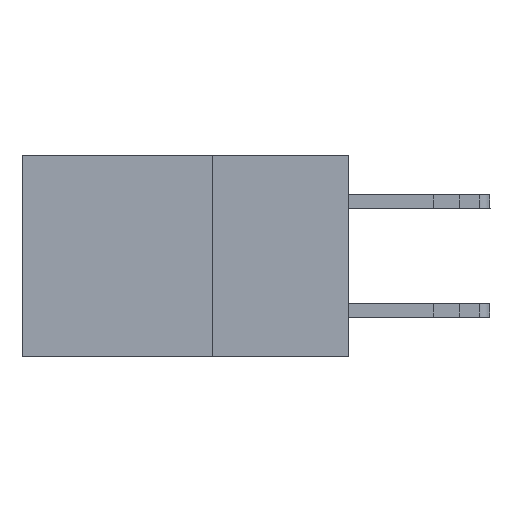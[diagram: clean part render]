
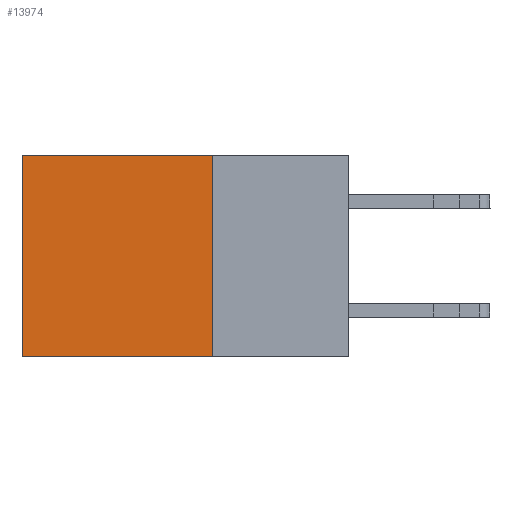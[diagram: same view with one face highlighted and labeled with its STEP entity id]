
A CAD part, left-side view. The second image highlights one B-rep face of the part: STEP entity #13974.
In plain terms, the highlighted planar face has unit normal (-1, 0, 0).
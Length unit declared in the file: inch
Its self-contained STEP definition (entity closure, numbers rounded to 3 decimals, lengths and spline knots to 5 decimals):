
#588 = FACE_OUTER_BOUND ( 'NONE', #6621, .T. ) ;
#638 = CARTESIAN_POINT ( 'NONE',  ( 0.2615, 0.25, -0.37 ) ) ;
#677 = VERTEX_POINT ( 'NONE', #7158 ) ;
#799 = DIRECTION ( 'NONE',  ( 0., 1., 0. ) ) ;
#973 = VECTOR ( 'NONE', #9903, 39.37008 ) ;
#1036 = VERTEX_POINT ( 'NONE', #10401 ) ;
#1216 = VERTEX_POINT ( 'NONE', #12001 ) ;
#2513 = DIRECTION ( 'NONE',  ( 0., 0., -1. ) ) ;
#3322 = ORIENTED_EDGE ( 'NONE', *, *, #8319, .T. ) ;
#3716 = CARTESIAN_POINT ( 'NONE',  ( 0.2615, 0.25, -0.37 ) ) ;
#4229 = DIRECTION ( 'NONE',  ( 0., 1., 0. ) ) ;
#4255 = PLANE ( 'NONE',  #14302 ) ;
#4331 = VECTOR ( 'NONE', #4229, 39.37008 ) ;
#5989 = DIRECTION ( 'NONE',  ( 1., 0., 0. ) ) ;
#6621 = EDGE_LOOP ( 'NONE', ( #3322, #10829, #8541, #14708 ) ) ;
#7143 = LINE ( 'NONE', #3716, #9601 ) ;
#7158 = CARTESIAN_POINT ( 'NONE',  ( 0.2615, 0.6, 0. ) ) ;
#7565 = EDGE_CURVE ( 'NONE', #1036, #677, #15465, .T. ) ;
#7745 = LINE ( 'NONE', #11075, #973 ) ;
#7945 = CARTESIAN_POINT ( 'NONE',  ( 0.2615, 0.25, 0. ) ) ;
#8283 = EDGE_CURVE ( 'NONE', #1036, #13967, #7143, .T. ) ;
#8319 = EDGE_CURVE ( 'NONE', #677, #1216, #7745, .T. ) ;
#8541 = ORIENTED_EDGE ( 'NONE', *, *, #8283, .F. ) ;
#9601 = VECTOR ( 'NONE', #2513, 39.37008 ) ;
#9903 = DIRECTION ( 'NONE',  ( 0., 0., -1. ) ) ;
#10112 = VECTOR ( 'NONE', #799, 39.37008 ) ;
#10401 = CARTESIAN_POINT ( 'NONE',  ( 0.2615, 0.25, 0. ) ) ;
#10534 = EDGE_CURVE ( 'NONE', #13967, #1216, #11694, .T. ) ;
#10829 = ORIENTED_EDGE ( 'NONE', *, *, #10534, .F. ) ;
#10980 = DIRECTION ( 'NONE',  ( 0., 0., -1. ) ) ;
#11075 = CARTESIAN_POINT ( 'NONE',  ( 0.2615, 0.6, -0.37 ) ) ;
#11694 = LINE ( 'NONE', #638, #4331 ) ;
#11719 = CARTESIAN_POINT ( 'NONE',  ( 0.2615, 0.25, -0.37 ) ) ;
#12001 = CARTESIAN_POINT ( 'NONE',  ( 0.2615, 0.6, -0.37 ) ) ;
#13909 = CARTESIAN_POINT ( 'NONE',  ( 0.2615, 0.25, -0.37 ) ) ;
#13967 = VERTEX_POINT ( 'NONE', #11719 ) ;
#13974 = ADVANCED_FACE ( 'NONE', ( #588 ), #4255, .F. ) ;
#14302 = AXIS2_PLACEMENT_3D ( 'NONE', #13909, #5989, #10980 ) ;
#14708 = ORIENTED_EDGE ( 'NONE', *, *, #7565, .T. ) ;
#15465 = LINE ( 'NONE', #7945, #10112 ) ;
